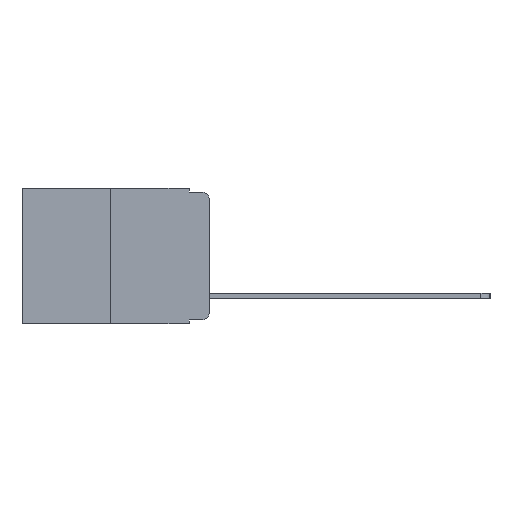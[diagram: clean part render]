
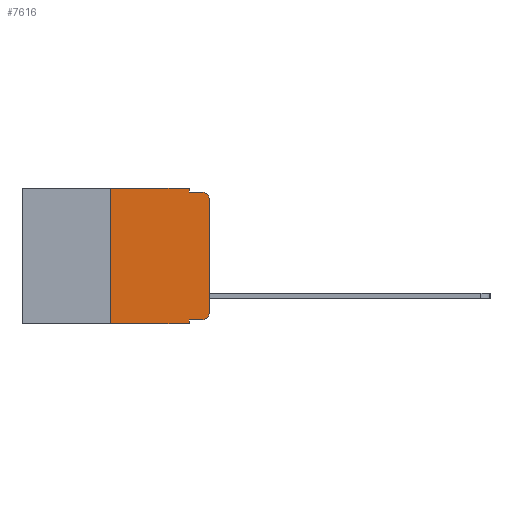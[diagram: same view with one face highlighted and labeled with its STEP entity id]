
A CAD part, left-side view. The second image highlights one B-rep face of the part: STEP entity #7616.
In plain terms, the highlighted planar face has unit normal (-1, 0, 0).
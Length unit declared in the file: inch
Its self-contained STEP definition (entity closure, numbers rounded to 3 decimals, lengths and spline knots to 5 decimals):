
#600 = CIRCLE ( 'NONE', #2399, 0.02 ) ;
#857 = CARTESIAN_POINT ( 'NONE',  ( 0., 0.051, -0.333 ) ) ;
#974 = DIRECTION ( 'NONE',  ( -1., 0., 0. ) ) ;
#1344 = VERTEX_POINT ( 'NONE', #6133 ) ;
#1796 = CARTESIAN_POINT ( 'NONE',  ( 0., 0.051, 0. ) ) ;
#2088 = LINE ( 'NONE', #3137, #10613 ) ;
#2399 = AXIS2_PLACEMENT_3D ( 'NONE', #8127, #974, #9271 ) ;
#3137 = CARTESIAN_POINT ( 'NONE',  ( 0., 0.051, -0.01 ) ) ;
#3242 = VERTEX_POINT ( 'NONE', #4970 ) ;
#3438 = LINE ( 'NONE', #10760, #12135 ) ;
#3911 = DIRECTION ( 'NONE',  ( 0., 0., -1. ) ) ;
#4013 = EDGE_CURVE ( 'NONE', #1344, #13755, #10602, .T. ) ;
#4173 = ORIENTED_EDGE ( 'NONE', *, *, #6946, .T. ) ;
#4289 = CARTESIAN_POINT ( 'NONE',  ( 0., 0.25, 0. ) ) ;
#4299 = PLANE ( 'NONE',  #12901 ) ;
#4358 = DIRECTION ( 'NONE',  ( 0., -1., 0. ) ) ;
#4695 = VECTOR ( 'NONE', #10246, 39.37008 ) ;
#4970 = CARTESIAN_POINT ( 'NONE',  ( 0., 0.25, 0. ) ) ;
#5465 = DIRECTION ( 'NONE',  ( 0., 0., 1. ) ) ;
#5478 = DIRECTION ( 'NONE',  ( 0., 0., -1. ) ) ;
#5508 = LINE ( 'NONE', #4289, #8573 ) ;
#5654 = VERTEX_POINT ( 'NONE', #1796 ) ;
#5805 = EDGE_CURVE ( 'NONE', #3242, #5654, #7736, .T. ) ;
#5819 = CARTESIAN_POINT ( 'NONE',  ( 0., 0.051, -0.333 ) ) ;
#6133 = CARTESIAN_POINT ( 'NONE',  ( 0., 0.25, -0.343 ) ) ;
#6191 = EDGE_CURVE ( 'NONE', #7907, #8148, #11736, .T. ) ;
#6340 = EDGE_LOOP ( 'NONE', ( #6843, #9828, #11454, #14732, #6563, #12472, #6919, #12831, #4173, #13165 ) ) ;
#6501 = DIRECTION ( 'NONE',  ( -1., 0., 0. ) ) ;
#6563 = ORIENTED_EDGE ( 'NONE', *, *, #5805, .F. ) ;
#6843 = ORIENTED_EDGE ( 'NONE', *, *, #14390, .T. ) ;
#6919 = ORIENTED_EDGE ( 'NONE', *, *, #4013, .T. ) ;
#6946 = EDGE_CURVE ( 'NONE', #12776, #7907, #7534, .T. ) ;
#7509 = DIRECTION ( 'NONE',  ( 0., -1., 0. ) ) ;
#7526 = VERTEX_POINT ( 'NONE', #9808 ) ;
#7534 = LINE ( 'NONE', #857, #9822 ) ;
#7579 = AXIS2_PLACEMENT_3D ( 'NONE', #13151, #6501, #14280 ) ;
#7599 = VECTOR ( 'NONE', #7509, 39.37008 ) ;
#7616 = ADVANCED_FACE ( 'NONE', ( #12900 ), #4299, .F. ) ;
#7679 = EDGE_CURVE ( 'NONE', #12776, #13755, #11855, .T. ) ;
#7736 = LINE ( 'NONE', #11348, #4695 ) ;
#7907 = VERTEX_POINT ( 'NONE', #14812 ) ;
#8085 = VECTOR ( 'NONE', #10545, 39.37008 ) ;
#8127 = CARTESIAN_POINT ( 'NONE',  ( 0., 0.02, -0.03 ) ) ;
#8148 = VERTEX_POINT ( 'NONE', #10916 ) ;
#8471 = CARTESIAN_POINT ( 'NONE',  ( 0., 0., -0.03 ) ) ;
#8573 = VECTOR ( 'NONE', #5465, 39.37008 ) ;
#9271 = DIRECTION ( 'NONE',  ( 0., 0., -1. ) ) ;
#9307 = VECTOR ( 'NONE', #14528, 39.37008 ) ;
#9808 = CARTESIAN_POINT ( 'NONE',  ( 0., 0.02, -0.01 ) ) ;
#9822 = VECTOR ( 'NONE', #10260, 39.37008 ) ;
#9828 = ORIENTED_EDGE ( 'NONE', *, *, #13652, .T. ) ;
#9957 = EDGE_CURVE ( 'NONE', #1344, #3242, #5508, .T. ) ;
#10246 = DIRECTION ( 'NONE',  ( 0., -1., 0. ) ) ;
#10260 = DIRECTION ( 'NONE',  ( 0., -1., 0. ) ) ;
#10545 = DIRECTION ( 'NONE',  ( 0., 0., 1. ) ) ;
#10602 = LINE ( 'NONE', #11915, #7599 ) ;
#10613 = VECTOR ( 'NONE', #4358, 39.37008 ) ;
#10711 = EDGE_CURVE ( 'NONE', #5654, #10779, #3438, .T. ) ;
#10760 = CARTESIAN_POINT ( 'NONE',  ( 0., 0.051, 0. ) ) ;
#10779 = VERTEX_POINT ( 'NONE', #14156 ) ;
#10916 = CARTESIAN_POINT ( 'NONE',  ( 0., 0., -0.313 ) ) ;
#11032 = LINE ( 'NONE', #14915, #8085 ) ;
#11106 = CARTESIAN_POINT ( 'NONE',  ( 0., 0.473, 0. ) ) ;
#11348 = CARTESIAN_POINT ( 'NONE',  ( 0., 0.473, 0. ) ) ;
#11430 = EDGE_CURVE ( 'NONE', #10779, #7526, #2088, .T. ) ;
#11454 = ORIENTED_EDGE ( 'NONE', *, *, #11430, .F. ) ;
#11736 = CIRCLE ( 'NONE', #7579, 0.02 ) ;
#11855 = LINE ( 'NONE', #13404, #9307 ) ;
#11915 = CARTESIAN_POINT ( 'NONE',  ( 0., 0.473, -0.343 ) ) ;
#12135 = VECTOR ( 'NONE', #3911, 39.37008 ) ;
#12185 = DIRECTION ( 'NONE',  ( 1., 0., 0. ) ) ;
#12472 = ORIENTED_EDGE ( 'NONE', *, *, #9957, .F. ) ;
#12664 = CARTESIAN_POINT ( 'NONE',  ( 0., 0.051, -0.343 ) ) ;
#12776 = VERTEX_POINT ( 'NONE', #5819 ) ;
#12831 = ORIENTED_EDGE ( 'NONE', *, *, #7679, .F. ) ;
#12900 = FACE_OUTER_BOUND ( 'NONE', #6340, .T. ) ;
#12901 = AXIS2_PLACEMENT_3D ( 'NONE', #11106, #12185, #5478 ) ;
#13151 = CARTESIAN_POINT ( 'NONE',  ( 0., 0.02, -0.313 ) ) ;
#13165 = ORIENTED_EDGE ( 'NONE', *, *, #6191, .T. ) ;
#13404 = CARTESIAN_POINT ( 'NONE',  ( 0., 0.051, 0. ) ) ;
#13652 = EDGE_CURVE ( 'NONE', #13872, #7526, #600, .T. ) ;
#13755 = VERTEX_POINT ( 'NONE', #12664 ) ;
#13872 = VERTEX_POINT ( 'NONE', #8471 ) ;
#14156 = CARTESIAN_POINT ( 'NONE',  ( 0., 0.051, -0.01 ) ) ;
#14280 = DIRECTION ( 'NONE',  ( 0., 0., -1. ) ) ;
#14390 = EDGE_CURVE ( 'NONE', #8148, #13872, #11032, .T. ) ;
#14528 = DIRECTION ( 'NONE',  ( 0., 0., -1. ) ) ;
#14732 = ORIENTED_EDGE ( 'NONE', *, *, #10711, .F. ) ;
#14812 = CARTESIAN_POINT ( 'NONE',  ( 0., 0.02, -0.333 ) ) ;
#14915 = CARTESIAN_POINT ( 'NONE',  ( 0., 0., 0. ) ) ;
